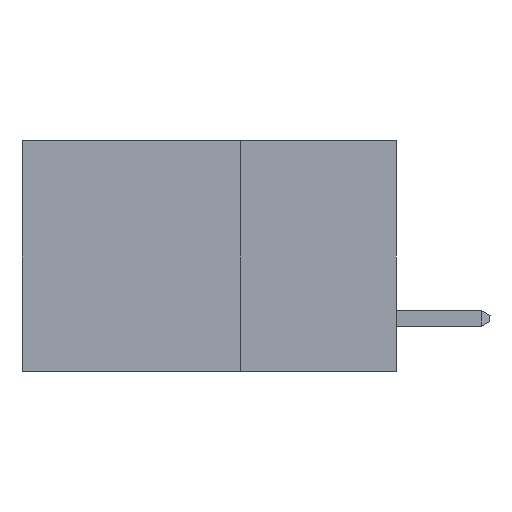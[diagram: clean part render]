
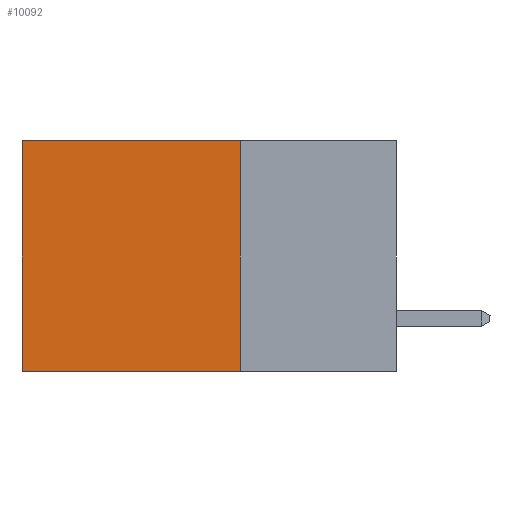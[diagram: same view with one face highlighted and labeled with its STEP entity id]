
A CAD part, left-side view. The second image highlights one B-rep face of the part: STEP entity #10092.
In plain terms, the highlighted planar face has unit normal (-1, 0, 0).
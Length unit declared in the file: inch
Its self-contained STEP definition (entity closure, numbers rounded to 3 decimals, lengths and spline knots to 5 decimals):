
#98 = CARTESIAN_POINT ( 'NONE',  ( 0.2615, 0.25, 0. ) ) ;
#562 = CARTESIAN_POINT ( 'NONE',  ( 0.2615, 0.25, -0.37 ) ) ;
#903 = VECTOR ( 'NONE', #11409, 39.37008 ) ;
#1001 = VERTEX_POINT ( 'NONE', #98 ) ;
#1528 = EDGE_LOOP ( 'NONE', ( #3433, #12008, #6790, #5060 ) ) ;
#2657 = CARTESIAN_POINT ( 'NONE',  ( 0.2615, 0.25, -0.37 ) ) ;
#3433 = ORIENTED_EDGE ( 'NONE', *, *, #3594, .T. ) ;
#3594 = EDGE_CURVE ( 'NONE', #8306, #11424, #7176, .T. ) ;
#3666 = PLANE ( 'NONE',  #7941 ) ;
#3756 = DIRECTION ( 'NONE',  ( 0., 1., 0. ) ) ;
#3895 = DIRECTION ( 'NONE',  ( 0., 1., 0. ) ) ;
#4385 = VECTOR ( 'NONE', #12532, 39.37008 ) ;
#4917 = CARTESIAN_POINT ( 'NONE',  ( 0.2615, 0.25, 0. ) ) ;
#5060 = ORIENTED_EDGE ( 'NONE', *, *, #13026, .T. ) ;
#5194 = CARTESIAN_POINT ( 'NONE',  ( 0.2615, 0.6, -0.37 ) ) ;
#5809 = EDGE_CURVE ( 'NONE', #1001, #12650, #12334, .T. ) ;
#6790 = ORIENTED_EDGE ( 'NONE', *, *, #5809, .F. ) ;
#6822 = DIRECTION ( 'NONE',  ( 1., 0., 0. ) ) ;
#7176 = LINE ( 'NONE', #5194, #903 ) ;
#7489 = CARTESIAN_POINT ( 'NONE',  ( 0.2615, 0.6, -0.37 ) ) ;
#7941 = AXIS2_PLACEMENT_3D ( 'NONE', #562, #6822, #11010 ) ;
#7977 = CARTESIAN_POINT ( 'NONE',  ( 0.2615, 0.6, 0. ) ) ;
#8306 = VERTEX_POINT ( 'NONE', #7977 ) ;
#8423 = VECTOR ( 'NONE', #3756, 39.37008 ) ;
#9090 = CARTESIAN_POINT ( 'NONE',  ( 0.2615, 0.25, -0.37 ) ) ;
#10092 = ADVANCED_FACE ( 'NONE', ( #13125 ), #3666, .F. ) ;
#11010 = DIRECTION ( 'NONE',  ( 0., 0., -1. ) ) ;
#11290 = EDGE_CURVE ( 'NONE', #12650, #11424, #13366, .T. ) ;
#11409 = DIRECTION ( 'NONE',  ( 0., 0., -1. ) ) ;
#11424 = VERTEX_POINT ( 'NONE', #7489 ) ;
#12008 = ORIENTED_EDGE ( 'NONE', *, *, #11290, .F. ) ;
#12334 = LINE ( 'NONE', #13461, #4385 ) ;
#12532 = DIRECTION ( 'NONE',  ( 0., 0., -1. ) ) ;
#12650 = VERTEX_POINT ( 'NONE', #9090 ) ;
#12835 = VECTOR ( 'NONE', #3895, 39.37008 ) ;
#13026 = EDGE_CURVE ( 'NONE', #1001, #8306, #13210, .T. ) ;
#13125 = FACE_OUTER_BOUND ( 'NONE', #1528, .T. ) ;
#13210 = LINE ( 'NONE', #4917, #8423 ) ;
#13366 = LINE ( 'NONE', #2657, #12835 ) ;
#13461 = CARTESIAN_POINT ( 'NONE',  ( 0.2615, 0.25, -0.37 ) ) ;
